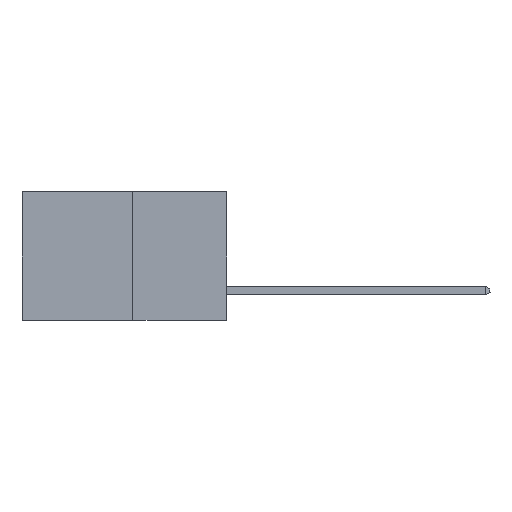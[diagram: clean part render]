
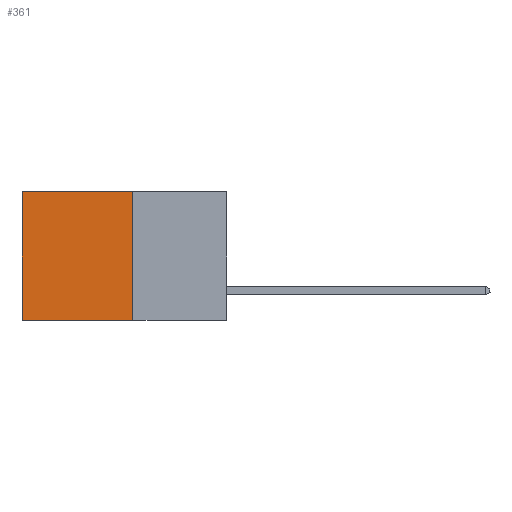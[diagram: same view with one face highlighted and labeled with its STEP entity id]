
A CAD part, left-side view. The second image highlights one B-rep face of the part: STEP entity #361.
In plain terms, the highlighted planar face has unit normal (-1, 0, 0).
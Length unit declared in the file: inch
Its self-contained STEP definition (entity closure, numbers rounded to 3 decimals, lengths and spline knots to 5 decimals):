
#361 = ADVANCED_FACE ( 'NONE', ( #6190 ), #7684, .F. ) ;
#640 = CARTESIAN_POINT ( 'NONE',  ( 0.277, 0.59, -0.37 ) ) ;
#918 = LINE ( 'NONE', #11000, #10104 ) ;
#1417 = VERTEX_POINT ( 'NONE', #640 ) ;
#1500 = ORIENTED_EDGE ( 'NONE', *, *, #3653, .T. ) ;
#1576 = ORIENTED_EDGE ( 'NONE', *, *, #6221, .F. ) ;
#1730 = ORIENTED_EDGE ( 'NONE', *, *, #6315, .F. ) ;
#1853 = ORIENTED_EDGE ( 'NONE', *, *, #3321, .T. ) ;
#2082 = DIRECTION ( 'NONE',  ( 0., 0., -1. ) ) ;
#2763 = LINE ( 'NONE', #8766, #5629 ) ;
#2772 = VECTOR ( 'NONE', #4799, 39.37008 ) ;
#2908 = CARTESIAN_POINT ( 'NONE',  ( 0.277, 0.27, -0.37 ) ) ;
#2994 = EDGE_LOOP ( 'NONE', ( #1500, #1576, #1730, #1853 ) ) ;
#3270 = VERTEX_POINT ( 'NONE', #6773 ) ;
#3321 = EDGE_CURVE ( 'NONE', #3270, #7799, #9166, .T. ) ;
#3653 = EDGE_CURVE ( 'NONE', #7799, #1417, #2763, .T. ) ;
#4602 = VECTOR ( 'NONE', #2082, 39.37008 ) ;
#4799 = DIRECTION ( 'NONE',  ( 0., 1., 0. ) ) ;
#5052 = CARTESIAN_POINT ( 'NONE',  ( 0.277, 0.27, 0. ) ) ;
#5629 = VECTOR ( 'NONE', #9532, 39.37008 ) ;
#6190 = FACE_OUTER_BOUND ( 'NONE', #2994, .T. ) ;
#6221 = EDGE_CURVE ( 'NONE', #7722, #1417, #918, .T. ) ;
#6315 = EDGE_CURVE ( 'NONE', #3270, #7722, #10913, .T. ) ;
#6773 = CARTESIAN_POINT ( 'NONE',  ( 0.277, 0.27, 0. ) ) ;
#6942 = DIRECTION ( 'NONE',  ( 1., 0., 0. ) ) ;
#7223 = DIRECTION ( 'NONE',  ( 0., 1., 0. ) ) ;
#7671 = AXIS2_PLACEMENT_3D ( 'NONE', #10276, #6942, #9347 ) ;
#7684 = PLANE ( 'NONE',  #7671 ) ;
#7722 = VERTEX_POINT ( 'NONE', #2908 ) ;
#7799 = VERTEX_POINT ( 'NONE', #8835 ) ;
#8766 = CARTESIAN_POINT ( 'NONE',  ( 0.277, 0.59, -0.37 ) ) ;
#8835 = CARTESIAN_POINT ( 'NONE',  ( 0.277, 0.59, 0. ) ) ;
#9166 = LINE ( 'NONE', #5052, #2772 ) ;
#9347 = DIRECTION ( 'NONE',  ( 0., 0., -1. ) ) ;
#9532 = DIRECTION ( 'NONE',  ( 0., 0., -1. ) ) ;
#9598 = CARTESIAN_POINT ( 'NONE',  ( 0.277, 0.27, -0.37 ) ) ;
#10104 = VECTOR ( 'NONE', #7223, 39.37008 ) ;
#10276 = CARTESIAN_POINT ( 'NONE',  ( 0.277, 0.27, -0.37 ) ) ;
#10913 = LINE ( 'NONE', #9598, #4602 ) ;
#11000 = CARTESIAN_POINT ( 'NONE',  ( 0.277, 0.27, -0.37 ) ) ;
